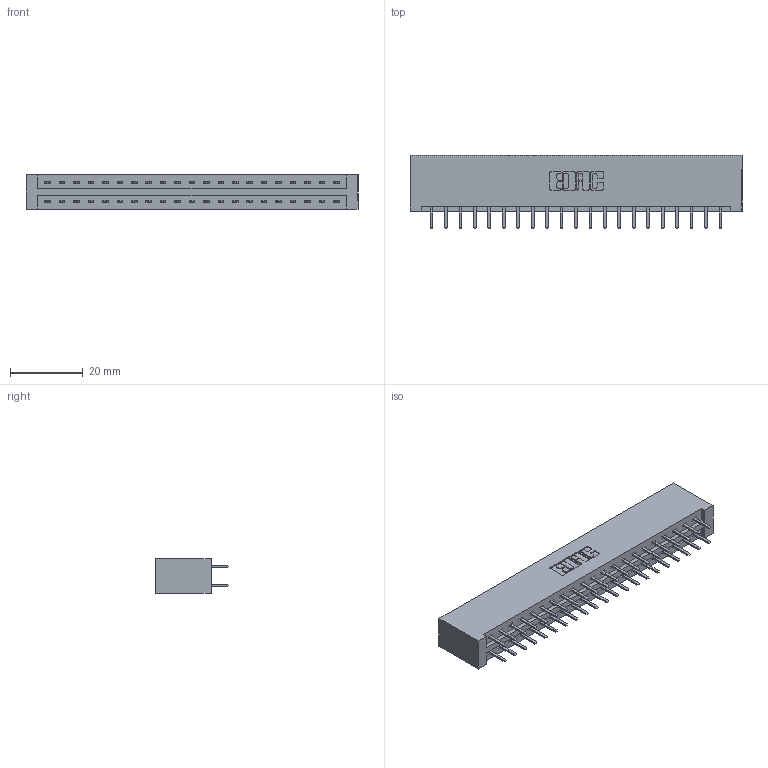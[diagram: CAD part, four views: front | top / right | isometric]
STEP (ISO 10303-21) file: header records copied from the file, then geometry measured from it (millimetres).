
FILE_DESCRIPTION (( 'STEP AP203' ), '1' );
FILE_NAME ('387-042-520-201.STEP', '2018-09-19T21:29:08', ( '' ), ( '' ), 'SwSTEP 2.0', 'SolidWorks 2016', '' );
FILE_SCHEMA (( 'CONFIG_CONTROL_DESIGN' ));
Length unit declared in the file: inch
Products named in the file (3): 337 Part_No Mounting Lugs; 345-292-001_345-293-120; 387-042-520-201
Assembly tree (43 placements, depth 2):
  387-042-520-201
    337 Part_No Mounting Lugs
    345-292-001_345-293-120  x42
Bounding box: 91.08 x 20.02 x 9.4 mm (x, y, z)
Volume: 10061.9 mm3; surface area: 11174.5 mm2
Topology: 43 solids, 43 shells, 2542 faces, 7385 edges, 4810 vertices
Faces by surface type: plane 1746, cylinder 796
Entity records: 18835 total; most frequent: CARTESIAN_POINT 3202, ORIENTED_EDGE 3126, DIRECTION 2743, EDGE_CURVE 1563, VECTOR 1439, LINE 1439, VERTEX_POINT 1038, AXIS2_PLACEMENT_3D 652
